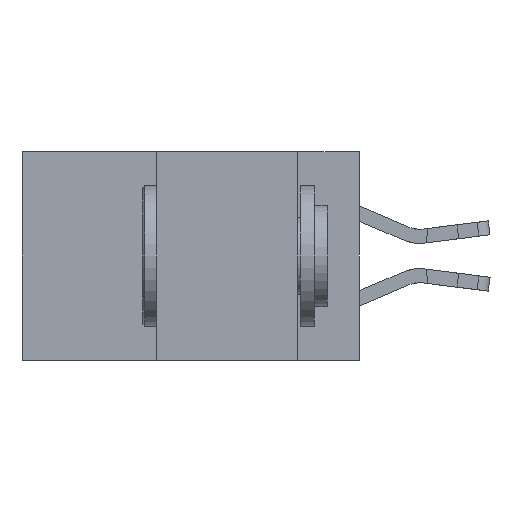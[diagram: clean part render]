
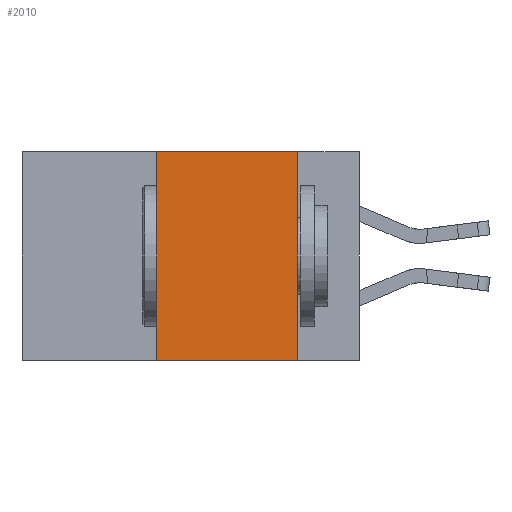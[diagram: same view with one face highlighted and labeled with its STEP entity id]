
A CAD part, left-side view. The second image highlights one B-rep face of the part: STEP entity #2010.
In plain terms, the highlighted planar face has unit normal (-1, 0, 0).
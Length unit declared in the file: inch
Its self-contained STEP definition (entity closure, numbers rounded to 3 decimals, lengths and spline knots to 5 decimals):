
#751 = CARTESIAN_POINT ( 'NONE',  ( 0., 0.36, 0. ) ) ;
#993 = VECTOR ( 'NONE', #14792, 39.37008 ) ;
#1054 = AXIS2_PLACEMENT_3D ( 'NONE', #7600, #18185, #21915 ) ;
#2010 = ADVANCED_FACE ( 'NONE', ( #21173 ), #20125, .F. ) ;
#2716 = VERTEX_POINT ( 'NONE', #2989 ) ;
#2989 = CARTESIAN_POINT ( 'NONE',  ( 0., 0.11, 0. ) ) ;
#3004 = ORIENTED_EDGE ( 'NONE', *, *, #12279, .F. ) ;
#3018 = VECTOR ( 'NONE', #13129, 39.37008 ) ;
#3368 = VERTEX_POINT ( 'NONE', #20642 ) ;
#4030 = EDGE_CURVE ( 'NONE', #12986, #21954, #5708, .T. ) ;
#4136 = EDGE_LOOP ( 'NONE', ( #3004, #15041, #20088, #6676 ) ) ;
#4822 = EDGE_CURVE ( 'NONE', #21954, #2716, #5946, .T. ) ;
#5402 = CARTESIAN_POINT ( 'NONE',  ( 0., 0.11, 0. ) ) ;
#5708 = LINE ( 'NONE', #751, #993 ) ;
#5910 = DIRECTION ( 'NONE',  ( 0., -1., 0. ) ) ;
#5946 = LINE ( 'NONE', #16422, #10672 ) ;
#6676 = ORIENTED_EDGE ( 'NONE', *, *, #9354, .T. ) ;
#7600 = CARTESIAN_POINT ( 'NONE',  ( 0., 0.6, 0. ) ) ;
#9066 = CARTESIAN_POINT ( 'NONE',  ( 0., 0.36, 0. ) ) ;
#9354 = EDGE_CURVE ( 'NONE', #12986, #3368, #22755, .T. ) ;
#10672 = VECTOR ( 'NONE', #5910, 39.37008 ) ;
#12237 = LINE ( 'NONE', #5402, #3018 ) ;
#12279 = EDGE_CURVE ( 'NONE', #2716, #3368, #12237, .T. ) ;
#12986 = VERTEX_POINT ( 'NONE', #21334 ) ;
#13129 = DIRECTION ( 'NONE',  ( 0., 0., -1. ) ) ;
#13901 = VECTOR ( 'NONE', #22989, 39.37008 ) ;
#14792 = DIRECTION ( 'NONE',  ( 0., 0., 1. ) ) ;
#15041 = ORIENTED_EDGE ( 'NONE', *, *, #4822, .F. ) ;
#16422 = CARTESIAN_POINT ( 'NONE',  ( 0., 0.6, 0. ) ) ;
#18185 = DIRECTION ( 'NONE',  ( 1., 0., 0. ) ) ;
#20088 = ORIENTED_EDGE ( 'NONE', *, *, #4030, .F. ) ;
#20125 = PLANE ( 'NONE',  #1054 ) ;
#20642 = CARTESIAN_POINT ( 'NONE',  ( 0., 0.11, -0.37 ) ) ;
#21173 = FACE_OUTER_BOUND ( 'NONE', #4136, .T. ) ;
#21334 = CARTESIAN_POINT ( 'NONE',  ( 0., 0.36, -0.37 ) ) ;
#21915 = DIRECTION ( 'NONE',  ( 0., 0., -1. ) ) ;
#21954 = VERTEX_POINT ( 'NONE', #9066 ) ;
#22755 = LINE ( 'NONE', #22914, #13901 ) ;
#22914 = CARTESIAN_POINT ( 'NONE',  ( 0., 0.6, -0.37 ) ) ;
#22989 = DIRECTION ( 'NONE',  ( 0., -1., 0. ) ) ;
